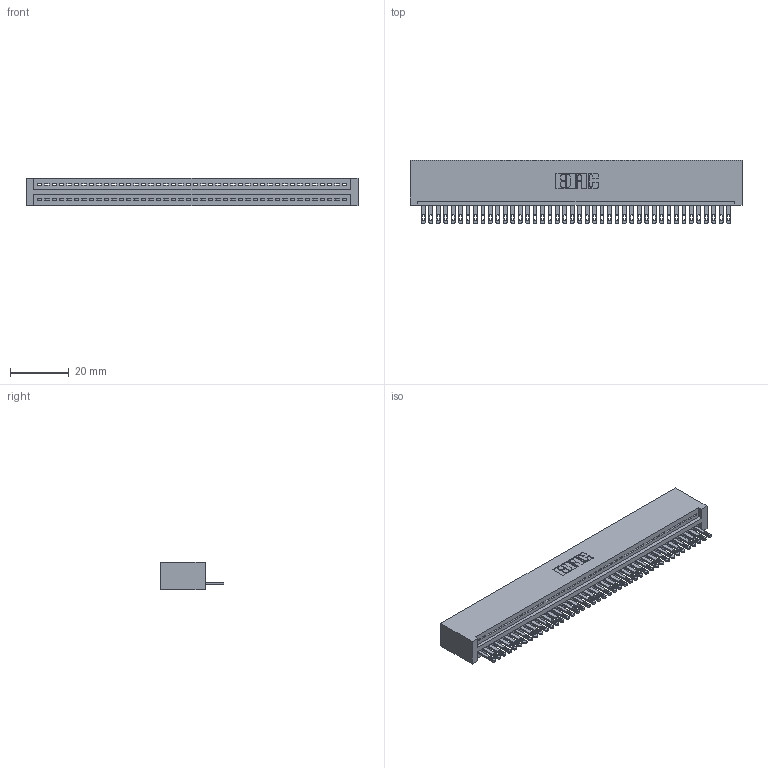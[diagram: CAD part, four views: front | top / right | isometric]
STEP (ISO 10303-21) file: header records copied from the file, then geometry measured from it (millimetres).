
FILE_DESCRIPTION (( 'STEP AP203' ), '1' );
FILE_NAME ('345-042-500-101.STEP', '2019-10-08T13:21:46', ( '' ), ( '' ), 'SwSTEP 2.0', 'SolidWorks 2016', '' );
FILE_SCHEMA (( 'CONFIG_CONTROL_DESIGN' ));
Length unit declared in the file: inch
Products named in the file (3): 345 Part_No Mounting Lugs; 345-042-500-101; 345-292-001_345-293-100
Assembly tree (43 placements, depth 2):
  345-042-500-101
    345 Part_No Mounting Lugs
    345-292-001_345-293-100  x42
Bounding box: 113.28 x 21.51 x 9.4 mm (x, y, z)
Volume: 11370.2 mm3; surface area: 15394.4 mm2
Topology: 43 solids, 43 shells, 2386 faces, 7373 edges, 4914 vertices
Faces by surface type: plane 1504, cylinder 882
Entity records: 31263 total; most frequent: CARTESIAN_POINT 5422, ORIENTED_EDGE 5398, DIRECTION 4731, EDGE_CURVE 2699, LINE 2403, VECTOR 2403, VERTEX_POINT 1798, AXIS2_PLACEMENT_3D 1164
